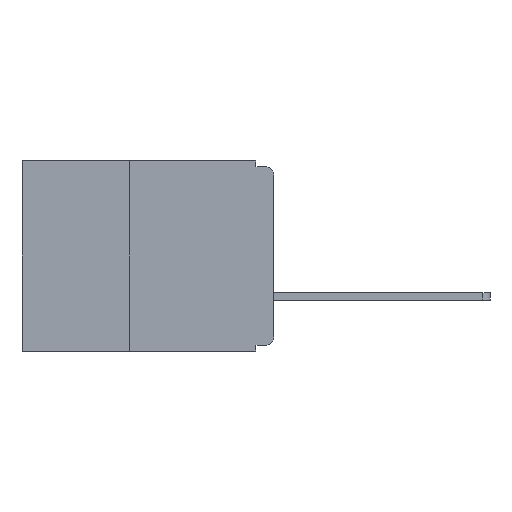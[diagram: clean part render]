
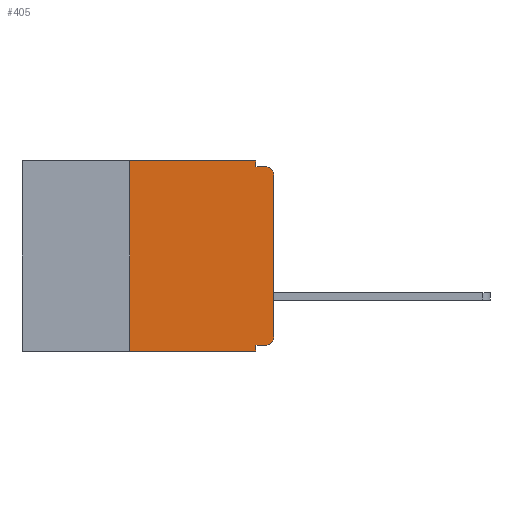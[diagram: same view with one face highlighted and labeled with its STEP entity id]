
A CAD part, left-side view. The second image highlights one B-rep face of the part: STEP entity #405.
In plain terms, the highlighted planar face has unit normal (-1, 0, 0).
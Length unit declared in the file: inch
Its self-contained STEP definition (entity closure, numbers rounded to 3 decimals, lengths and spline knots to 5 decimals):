
#211 = DIRECTION ( 'NONE',  ( -1., 0., 0. ) ) ;
#371 = EDGE_CURVE ( 'NONE', #16500, #14630, #17116, .T. ) ;
#405 = ADVANCED_FACE ( 'NONE', ( #3206 ), #21081, .F. ) ;
#1445 = EDGE_LOOP ( 'NONE', ( #18515, #23822, #15080, #29543, #4317, #23545, #29989, #24340, #6307, #23268 ) ) ;
#2143 = CARTESIAN_POINT ( 'NONE',  ( 0., 0.031, -0.32 ) ) ;
#2159 = AXIS2_PLACEMENT_3D ( 'NONE', #15050, #211, #17556 ) ;
#2744 = VERTEX_POINT ( 'NONE', #22276 ) ;
#3206 = FACE_OUTER_BOUND ( 'NONE', #1445, .T. ) ;
#3456 = VECTOR ( 'NONE', #13295, 39.37008 ) ;
#3987 = VECTOR ( 'NONE', #11010, 39.37008 ) ;
#4317 = ORIENTED_EDGE ( 'NONE', *, *, #13748, .F. ) ;
#5211 = CARTESIAN_POINT ( 'NONE',  ( 0., 0.437, 0. ) ) ;
#5793 = VERTEX_POINT ( 'NONE', #2143 ) ;
#5849 = CARTESIAN_POINT ( 'NONE',  ( 0., 0.437, -0.33 ) ) ;
#6138 = DIRECTION ( 'NONE',  ( 0., -1., 0. ) ) ;
#6307 = ORIENTED_EDGE ( 'NONE', *, *, #26777, .F. ) ;
#6750 = EDGE_CURVE ( 'NONE', #5793, #2744, #10884, .T. ) ;
#6960 = VECTOR ( 'NONE', #24479, 39.37008 ) ;
#6961 = CARTESIAN_POINT ( 'NONE',  ( 0., 0.031, 0. ) ) ;
#7294 = EDGE_CURVE ( 'NONE', #29023, #27315, #16654, .T. ) ;
#7726 = CARTESIAN_POINT ( 'NONE',  ( 0., 0.25, -0.33 ) ) ;
#8251 = VECTOR ( 'NONE', #10617, 39.37008 ) ;
#8518 = CARTESIAN_POINT ( 'NONE',  ( 0., 0., -0.01 ) ) ;
#9377 = EDGE_CURVE ( 'NONE', #21643, #21524, #22979, .T. ) ;
#9797 = CARTESIAN_POINT ( 'NONE',  ( 0., 0., 0. ) ) ;
#10020 = LINE ( 'NONE', #5849, #3456 ) ;
#10617 = DIRECTION ( 'NONE',  ( 0., 1., 0. ) ) ;
#10884 = LINE ( 'NONE', #27613, #30317 ) ;
#11004 = AXIS2_PLACEMENT_3D ( 'NONE', #16988, #16980, #16912 ) ;
#11010 = DIRECTION ( 'NONE',  ( 0., 0., -1. ) ) ;
#11322 = CARTESIAN_POINT ( 'NONE',  ( 0., 0.015, -0.32 ) ) ;
#12222 = EDGE_CURVE ( 'NONE', #14630, #23659, #17175, .T. ) ;
#12654 = DIRECTION ( 'NONE',  ( 0., -1., 0. ) ) ;
#12766 = LINE ( 'NONE', #9797, #6960 ) ;
#13295 = DIRECTION ( 'NONE',  ( 0., -1., 0. ) ) ;
#13748 = EDGE_CURVE ( 'NONE', #21524, #16500, #25438, .T. ) ;
#13842 = DIRECTION ( 'NONE',  ( 0., 0., 1. ) ) ;
#14630 = VERTEX_POINT ( 'NONE', #16435 ) ;
#14780 = LINE ( 'NONE', #18065, #8251 ) ;
#15050 = CARTESIAN_POINT ( 'NONE',  ( 0., 0.015, -0.025 ) ) ;
#15080 = ORIENTED_EDGE ( 'NONE', *, *, #12222, .F. ) ;
#15477 = EDGE_CURVE ( 'NONE', #27315, #16821, #12766, .T. ) ;
#16435 = CARTESIAN_POINT ( 'NONE',  ( 0., 0.031, -0.01 ) ) ;
#16500 = VERTEX_POINT ( 'NONE', #18697 ) ;
#16654 = CIRCLE ( 'NONE', #11004, 0.015 ) ;
#16821 = VERTEX_POINT ( 'NONE', #22265 ) ;
#16912 = DIRECTION ( 'NONE',  ( 0., 0., -1. ) ) ;
#16980 = DIRECTION ( 'NONE',  ( -1., 0., 0. ) ) ;
#16988 = CARTESIAN_POINT ( 'NONE',  ( 0., 0.015, -0.305 ) ) ;
#17116 = LINE ( 'NONE', #6961, #3987 ) ;
#17175 = LINE ( 'NONE', #8518, #22892 ) ;
#17556 = DIRECTION ( 'NONE',  ( 0., 0., -1. ) ) ;
#18042 = VECTOR ( 'NONE', #13842, 39.37008 ) ;
#18065 = CARTESIAN_POINT ( 'NONE',  ( 0., 0., -0.32 ) ) ;
#18515 = ORIENTED_EDGE ( 'NONE', *, *, #15477, .T. ) ;
#18697 = CARTESIAN_POINT ( 'NONE',  ( 0., 0.031, 0. ) ) ;
#19583 = CARTESIAN_POINT ( 'NONE',  ( 0., 0.25, 0. ) ) ;
#20110 = CARTESIAN_POINT ( 'NONE',  ( 0., 0.437, 0. ) ) ;
#20176 = CARTESIAN_POINT ( 'NONE',  ( 0., 0.015, -0.01 ) ) ;
#20335 = DIRECTION ( 'NONE',  ( 1., 0., 0. ) ) ;
#21081 = PLANE ( 'NONE',  #27862 ) ;
#21524 = VERTEX_POINT ( 'NONE', #19583 ) ;
#21643 = VERTEX_POINT ( 'NONE', #7726 ) ;
#21856 = CIRCLE ( 'NONE', #2159, 0.015 ) ;
#22265 = CARTESIAN_POINT ( 'NONE',  ( 0., 0., -0.025 ) ) ;
#22276 = CARTESIAN_POINT ( 'NONE',  ( 0., 0.031, -0.33 ) ) ;
#22892 = VECTOR ( 'NONE', #6138, 39.37008 ) ;
#22979 = LINE ( 'NONE', #30840, #18042 ) ;
#23182 = EDGE_CURVE ( 'NONE', #21643, #2744, #10020, .T. ) ;
#23268 = ORIENTED_EDGE ( 'NONE', *, *, #7294, .T. ) ;
#23545 = ORIENTED_EDGE ( 'NONE', *, *, #9377, .F. ) ;
#23659 = VERTEX_POINT ( 'NONE', #20176 ) ;
#23822 = ORIENTED_EDGE ( 'NONE', *, *, #24244, .T. ) ;
#24244 = EDGE_CURVE ( 'NONE', #16821, #23659, #21856, .T. ) ;
#24340 = ORIENTED_EDGE ( 'NONE', *, *, #6750, .F. ) ;
#24479 = DIRECTION ( 'NONE',  ( 0., 0., 1. ) ) ;
#25077 = DIRECTION ( 'NONE',  ( 0., 0., -1. ) ) ;
#25438 = LINE ( 'NONE', #5211, #30327 ) ;
#26777 = EDGE_CURVE ( 'NONE', #29023, #5793, #14780, .T. ) ;
#27315 = VERTEX_POINT ( 'NONE', #29792 ) ;
#27583 = DIRECTION ( 'NONE',  ( 0., 0., -1. ) ) ;
#27613 = CARTESIAN_POINT ( 'NONE',  ( 0., 0.031, -0.33 ) ) ;
#27862 = AXIS2_PLACEMENT_3D ( 'NONE', #20110, #20335, #25077 ) ;
#29023 = VERTEX_POINT ( 'NONE', #11322 ) ;
#29543 = ORIENTED_EDGE ( 'NONE', *, *, #371, .F. ) ;
#29792 = CARTESIAN_POINT ( 'NONE',  ( 0., 0., -0.305 ) ) ;
#29989 = ORIENTED_EDGE ( 'NONE', *, *, #23182, .T. ) ;
#30317 = VECTOR ( 'NONE', #27583, 39.37008 ) ;
#30327 = VECTOR ( 'NONE', #12654, 39.37008 ) ;
#30840 = CARTESIAN_POINT ( 'NONE',  ( 0., 0.25, -0.33 ) ) ;
